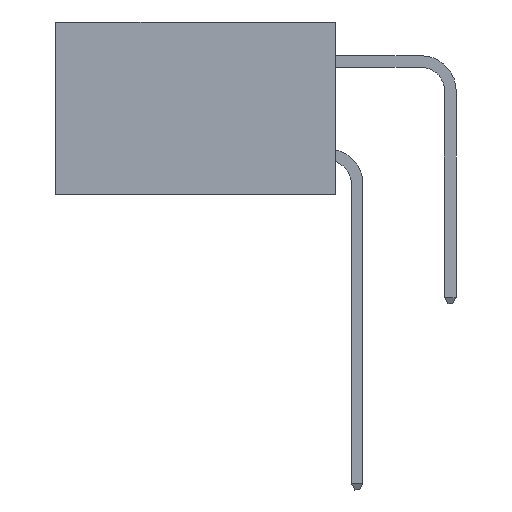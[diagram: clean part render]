
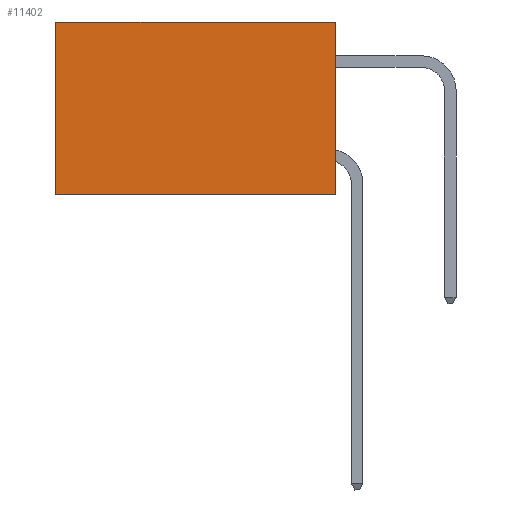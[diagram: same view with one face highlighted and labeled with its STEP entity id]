
A CAD part, left-side view. The second image highlights one B-rep face of the part: STEP entity #11402.
In plain terms, the highlighted planar face has unit normal (-1, 0, 0).
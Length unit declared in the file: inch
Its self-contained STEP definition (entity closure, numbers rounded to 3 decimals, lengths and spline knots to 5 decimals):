
#402 = DIRECTION ( 'NONE',  ( 0., 1., 0. ) ) ;
#485 = EDGE_CURVE ( 'NONE', #22874, #8820, #24495, .T. ) ;
#1274 = EDGE_CURVE ( 'NONE', #22874, #12073, #42494, .T. ) ;
#2620 = DIRECTION ( 'NONE',  ( 0., 1., 0. ) ) ;
#2945 = ORIENTED_EDGE ( 'NONE', *, *, #1274, .T. ) ;
#5427 = DIRECTION ( 'NONE',  ( 0., 0., -1. ) ) ;
#5618 = CARTESIAN_POINT ( 'NONE',  ( 0.2875, 0., 0. ) ) ;
#6670 = CARTESIAN_POINT ( 'NONE',  ( 0.2875, 0., 0. ) ) ;
#6718 = ORIENTED_EDGE ( 'NONE', *, *, #485, .F. ) ;
#7368 = AXIS2_PLACEMENT_3D ( 'NONE', #6670, #26842, #23450 ) ;
#8820 = VERTEX_POINT ( 'NONE', #38584 ) ;
#11158 = VECTOR ( 'NONE', #36418, 39.37008 ) ;
#11402 = ADVANCED_FACE ( 'NONE', ( #31045 ), #23605, .F. ) ;
#12073 = VERTEX_POINT ( 'NONE', #40383 ) ;
#12621 = CARTESIAN_POINT ( 'NONE',  ( 0.2875, 0.6, -0.37 ) ) ;
#13168 = CARTESIAN_POINT ( 'NONE',  ( 0.2875, 0., -0.37 ) ) ;
#13247 = EDGE_LOOP ( 'NONE', ( #30219, #22609, #6718, #2945 ) ) ;
#13736 = VECTOR ( 'NONE', #2620, 39.37008 ) ;
#14791 = LINE ( 'NONE', #13168, #13736 ) ;
#15136 = CARTESIAN_POINT ( 'NONE',  ( 0.2875, 0., 0. ) ) ;
#18654 = CARTESIAN_POINT ( 'NONE',  ( 0.2875, 0.6, 0. ) ) ;
#20522 = VECTOR ( 'NONE', #5427, 39.37008 ) ;
#22609 = ORIENTED_EDGE ( 'NONE', *, *, #25975, .F. ) ;
#22874 = VERTEX_POINT ( 'NONE', #15136 ) ;
#23178 = VERTEX_POINT ( 'NONE', #12621 ) ;
#23450 = DIRECTION ( 'NONE',  ( 0., 0., -1. ) ) ;
#23605 = PLANE ( 'NONE',  #7368 ) ;
#24495 = LINE ( 'NONE', #5618, #11158 ) ;
#25975 = EDGE_CURVE ( 'NONE', #8820, #23178, #14791, .T. ) ;
#26488 = VECTOR ( 'NONE', #402, 39.37008 ) ;
#26842 = DIRECTION ( 'NONE',  ( 1., 0., 0. ) ) ;
#30219 = ORIENTED_EDGE ( 'NONE', *, *, #32447, .T. ) ;
#30916 = CARTESIAN_POINT ( 'NONE',  ( 0.2875, 0., 0. ) ) ;
#31045 = FACE_OUTER_BOUND ( 'NONE', #13247, .T. ) ;
#32447 = EDGE_CURVE ( 'NONE', #12073, #23178, #42919, .T. ) ;
#36418 = DIRECTION ( 'NONE',  ( 0., 0., -1. ) ) ;
#38584 = CARTESIAN_POINT ( 'NONE',  ( 0.2875, 0., -0.37 ) ) ;
#40383 = CARTESIAN_POINT ( 'NONE',  ( 0.2875, 0.6, 0. ) ) ;
#42494 = LINE ( 'NONE', #30916, #26488 ) ;
#42919 = LINE ( 'NONE', #18654, #20522 ) ;
